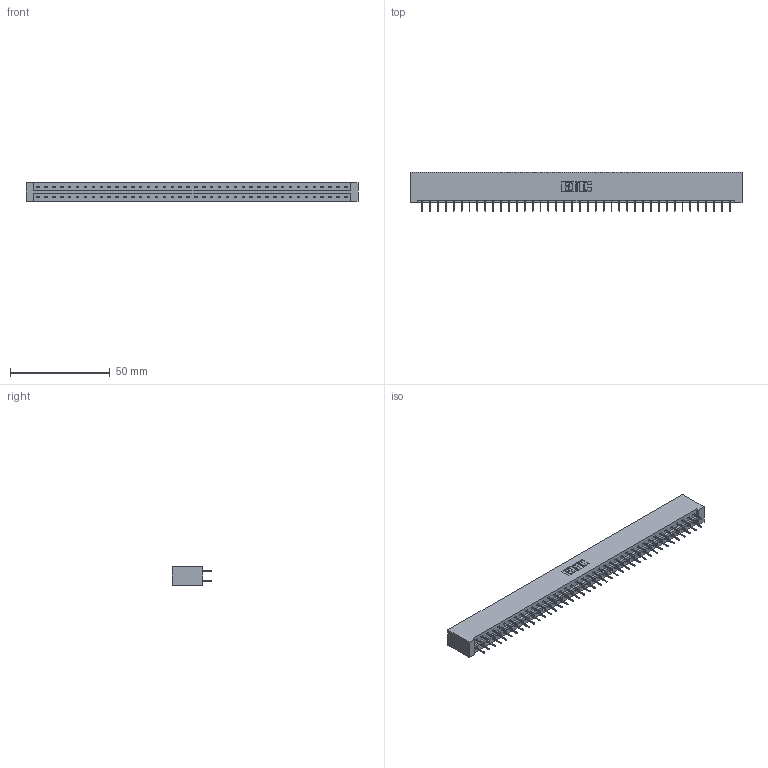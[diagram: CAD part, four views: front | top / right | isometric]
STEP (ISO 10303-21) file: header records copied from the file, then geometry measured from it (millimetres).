
FILE_DESCRIPTION (( 'STEP AP203' ), '1' );
FILE_NAME ('333-080-524-201.STEP', '2018-08-05T01:26:37', ( '' ), ( '' ), 'SwSTEP 2.0', 'SolidWorks 2016', '' );
FILE_SCHEMA (( 'CONFIG_CONTROL_DESIGN' ));
Length unit declared in the file: inch
Products named in the file (3): 345-292-001_345-293-124; 333-080-524-201; 333 Part_Lugless
Assembly tree (81 placements, depth 2):
  333-080-524-201
    333 Part_Lugless
    345-292-001_345-293-124  x80
Bounding box: 166.75 x 19.69 x 9.4 mm (x, y, z)
Volume: 17516.8 mm3; surface area: 20348.7 mm2
Topology: 81 solids, 81 shells, 4586 faces, 13007 edges, 8350 vertices
Faces by surface type: plane 3426, cylinder 1160
Entity records: 25789 total; most frequent: CARTESIAN_POINT 4274, ORIENTED_EDGE 4210, DIRECTION 3649, EDGE_CURVE 2105, VECTOR 1989, LINE 1989, VERTEX_POINT 1398, AXIS2_PLACEMENT_3D 830
